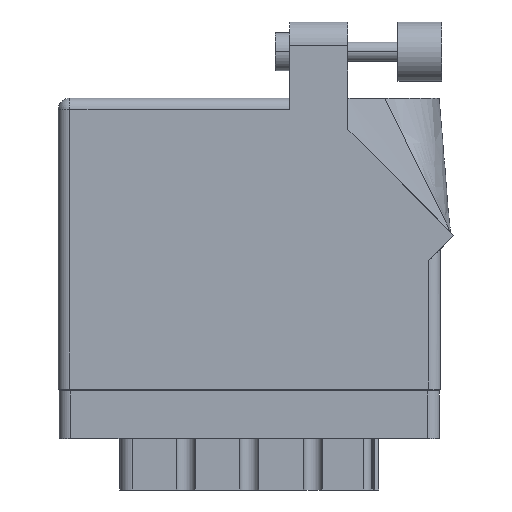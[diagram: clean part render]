
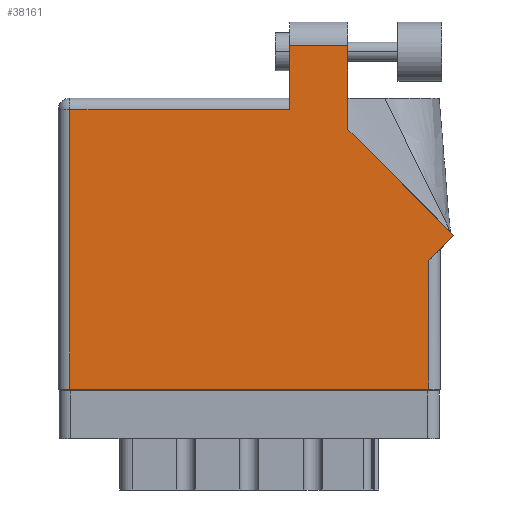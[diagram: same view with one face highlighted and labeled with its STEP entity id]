
A CAD part, front view. The second image highlights one B-rep face of the part: STEP entity #38161.
In plain terms, the highlighted face is planar.
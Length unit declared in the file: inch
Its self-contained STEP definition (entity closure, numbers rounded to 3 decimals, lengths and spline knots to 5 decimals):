
#27 = VERTEX_POINT ( 'NONE', #38444 ) ;
#81 = DIRECTION ( 'NONE',  ( 1., 0., 0. ) ) ;
#188 = EDGE_CURVE ( 'NONE', #13484, #22122, #34255, .T. ) ;
#1092 = CARTESIAN_POINT ( 'NONE',  ( 0.062, 0., 0. ) ) ;
#3277 = CARTESIAN_POINT ( 'NONE',  ( 1.524, 1.805, 0. ) ) ;
#3305 = CARTESIAN_POINT ( 'NONE',  ( 1.524, 1.36442, 0. ) ) ;
#6892 = CARTESIAN_POINT ( 'NONE',  ( 0., 0., 0. ) ) ;
#7288 = CARTESIAN_POINT ( 'NONE',  ( 1.524, 1.36442, 0. ) ) ;
#8503 = VECTOR ( 'NONE', #32656, 39.37008 ) ;
#8536 = VECTOR ( 'NONE', #29757, 39.37008 ) ;
#9131 = LINE ( 'NONE', #30630, #33472 ) ;
#10895 = VECTOR ( 'NONE', #30623, 39.37008 ) ;
#11043 = CARTESIAN_POINT ( 'NONE',  ( 0., 1.53, 0. ) ) ;
#11125 = ORIENTED_EDGE ( 'NONE', *, *, #22630, .T. ) ;
#11602 = DIRECTION ( 'NONE',  ( -1., 0., 0. ) ) ;
#11988 = EDGE_CURVE ( 'NONE', #36632, #26677, #36807, .T. ) ;
#13014 = EDGE_CURVE ( 'NONE', #35873, #20477, #40284, .T. ) ;
#13484 = VERTEX_POINT ( 'NONE', #36741 ) ;
#14248 = DIRECTION ( 'NONE',  ( 0., 0., -1. ) ) ;
#15500 = VERTEX_POINT ( 'NONE', #21572 ) ;
#16969 = LINE ( 'NONE', #36256, #8536 ) ;
#17601 = PLANE ( 'NONE',  #27728 ) ;
#17801 = CARTESIAN_POINT ( 'NONE',  ( 1.948, 0.737, 0. ) ) ;
#19777 = DIRECTION ( 'NONE',  ( 0., 1., 0. ) ) ;
#20477 = VERTEX_POINT ( 'NONE', #3277 ) ;
#20489 = CARTESIAN_POINT ( 'NONE',  ( 0.062, 1.468, 0. ) ) ;
#20512 = EDGE_CURVE ( 'NONE', #15500, #27, #29871, .T. ) ;
#20825 = ORIENTED_EDGE ( 'NONE', *, *, #20512, .T. ) ;
#21572 = CARTESIAN_POINT ( 'NONE',  ( 0.062, 0., 0. ) ) ;
#21706 = CARTESIAN_POINT ( 'NONE',  ( 1.217, 1.468, 0. ) ) ;
#22122 = VERTEX_POINT ( 'NONE', #27434 ) ;
#22630 = EDGE_CURVE ( 'NONE', #27, #13484, #29758, .T. ) ;
#24098 = ORIENTED_EDGE ( 'NONE', *, *, #31531, .T. ) ;
#24408 = VECTOR ( 'NONE', #40414, 39.37008 ) ;
#24961 = EDGE_CURVE ( 'NONE', #29402, #15500, #26363, .T. ) ;
#25862 = CARTESIAN_POINT ( 'NONE',  ( 2.08071, 0.80771, 0. ) ) ;
#26363 = LINE ( 'NONE', #1092, #8503 ) ;
#26677 = VERTEX_POINT ( 'NONE', #21706 ) ;
#27434 = CARTESIAN_POINT ( 'NONE',  ( 2.08071, 0.80771, 0. ) ) ;
#27728 = AXIS2_PLACEMENT_3D ( 'NONE', #11043, #14248, #11602 ) ;
#27776 = VECTOR ( 'NONE', #34160, 39.37008 ) ;
#28561 = CARTESIAN_POINT ( 'NONE',  ( 1.217, 1.805, 0. ) ) ;
#28854 = ORIENTED_EDGE ( 'NONE', *, *, #188, .T. ) ;
#29073 = DIRECTION ( 'NONE',  ( -1., 0., 0. ) ) ;
#29402 = VERTEX_POINT ( 'NONE', #20489 ) ;
#29645 = EDGE_CURVE ( 'NONE', #26677, #29402, #9131, .T. ) ;
#29757 = DIRECTION ( 'NONE',  ( -1., 0., 0. ) ) ;
#29758 = LINE ( 'NONE', #17801, #27776 ) ;
#29871 = LINE ( 'NONE', #6892, #35823 ) ;
#30538 = ORIENTED_EDGE ( 'NONE', *, *, #13014, .T. ) ;
#30623 = DIRECTION ( 'NONE',  ( 0.707, 0.707, 0. ) ) ;
#30630 = CARTESIAN_POINT ( 'NONE',  ( 0., 1.468, 0. ) ) ;
#31091 = CARTESIAN_POINT ( 'NONE',  ( 1.217, 1.53, 0. ) ) ;
#31290 = VECTOR ( 'NONE', #19777, 39.37008 ) ;
#31531 = EDGE_CURVE ( 'NONE', #22122, #35873, #36654, .T. ) ;
#31689 = VECTOR ( 'NONE', #35280, 39.37008 ) ;
#32656 = DIRECTION ( 'NONE',  ( 0., -1., 0. ) ) ;
#32830 = CARTESIAN_POINT ( 'NONE',  ( 2.01, 0.737, 0. ) ) ;
#33134 = EDGE_LOOP ( 'NONE', ( #30538, #39368, #38555, #36228, #37828, #20825, #11125, #28854, #24098 ) ) ;
#33472 = VECTOR ( 'NONE', #29073, 39.37008 ) ;
#34160 = DIRECTION ( 'NONE',  ( 0., 1., 0. ) ) ;
#34255 = LINE ( 'NONE', #32830, #10895 ) ;
#34505 = FACE_OUTER_BOUND ( 'NONE', #33134, .T. ) ;
#35280 = DIRECTION ( 'NONE',  ( -0.707, 0.707, 0. ) ) ;
#35823 = VECTOR ( 'NONE', #81, 39.37008 ) ;
#35873 = VERTEX_POINT ( 'NONE', #3305 ) ;
#36228 = ORIENTED_EDGE ( 'NONE', *, *, #29645, .T. ) ;
#36256 = CARTESIAN_POINT ( 'NONE',  ( 1.217, 1.805, 0. ) ) ;
#36632 = VERTEX_POINT ( 'NONE', #28561 ) ;
#36654 = LINE ( 'NONE', #25862, #31689 ) ;
#36741 = CARTESIAN_POINT ( 'NONE',  ( 1.948, 0.675, 0. ) ) ;
#36807 = LINE ( 'NONE', #31091, #24408 ) ;
#37828 = ORIENTED_EDGE ( 'NONE', *, *, #24961, .T. ) ;
#38161 = ADVANCED_FACE ( 'NONE', ( #34505 ), #17601, .F. ) ;
#38444 = CARTESIAN_POINT ( 'NONE',  ( 1.948, 0., 0. ) ) ;
#38555 = ORIENTED_EDGE ( 'NONE', *, *, #11988, .T. ) ;
#38654 = EDGE_CURVE ( 'NONE', #20477, #36632, #16969, .T. ) ;
#39368 = ORIENTED_EDGE ( 'NONE', *, *, #38654, .T. ) ;
#40284 = LINE ( 'NONE', #7288, #31290 ) ;
#40414 = DIRECTION ( 'NONE',  ( 0., -1., 0. ) ) ;
